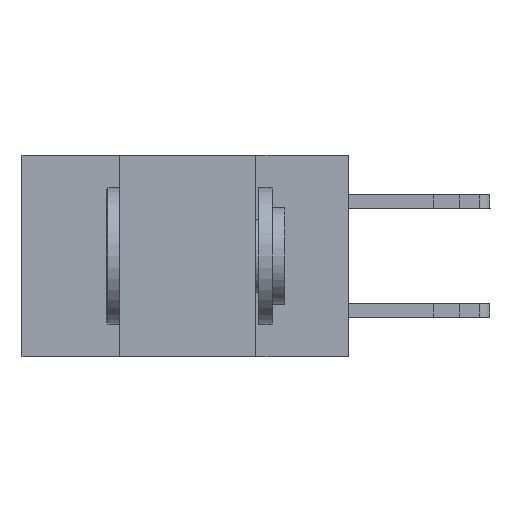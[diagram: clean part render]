
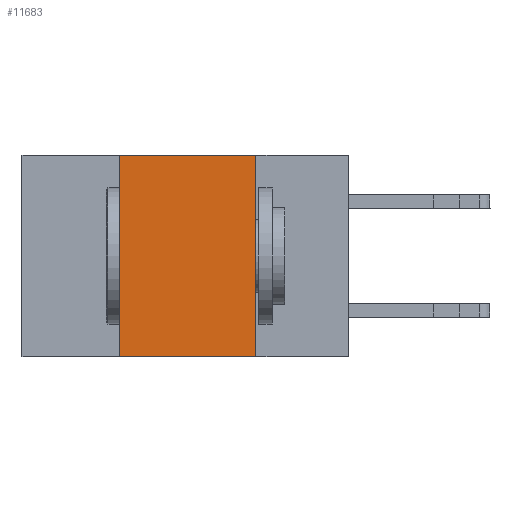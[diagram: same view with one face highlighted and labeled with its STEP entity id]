
A CAD part, left-side view. The second image highlights one B-rep face of the part: STEP entity #11683.
In plain terms, the highlighted planar face has unit normal (-1, 0, 0).
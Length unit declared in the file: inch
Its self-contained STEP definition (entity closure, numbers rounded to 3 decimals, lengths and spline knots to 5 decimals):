
#352 = ORIENTED_EDGE ( 'NONE', *, *, #7029, .T. ) ;
#1140 = CARTESIAN_POINT ( 'NONE',  ( 0., 0.42, -0.37 ) ) ;
#1278 = DIRECTION ( 'NONE',  ( 1., 0., 0. ) ) ;
#1381 = ORIENTED_EDGE ( 'NONE', *, *, #2035, .F. ) ;
#1482 = DIRECTION ( 'NONE',  ( 0., -1., 0. ) ) ;
#1679 = CARTESIAN_POINT ( 'NONE',  ( 0., 0.42, 0. ) ) ;
#1920 = LINE ( 'NONE', #9378, #4436 ) ;
#1985 = DIRECTION ( 'NONE',  ( 0., 0., -1. ) ) ;
#2035 = EDGE_CURVE ( 'NONE', #7792, #5594, #10503, .T. ) ;
#2076 = CARTESIAN_POINT ( 'NONE',  ( 0., 0.17, 0. ) ) ;
#2214 = AXIS2_PLACEMENT_3D ( 'NONE', #6106, #1278, #11693 ) ;
#2642 = VERTEX_POINT ( 'NONE', #2076 ) ;
#3270 = ORIENTED_EDGE ( 'NONE', *, *, #6280, .F. ) ;
#3851 = LINE ( 'NONE', #3910, #9724 ) ;
#3910 = CARTESIAN_POINT ( 'NONE',  ( 0., 0.6, -0.37 ) ) ;
#3925 = VECTOR ( 'NONE', #1482, 39.37008 ) ;
#4041 = EDGE_LOOP ( 'NONE', ( #8827, #3270, #1381, #352 ) ) ;
#4187 = FACE_OUTER_BOUND ( 'NONE', #4041, .T. ) ;
#4194 = LINE ( 'NONE', #5208, #3925 ) ;
#4436 = VECTOR ( 'NONE', #1985, 39.37008 ) ;
#5208 = CARTESIAN_POINT ( 'NONE',  ( 0., 0.6, 0. ) ) ;
#5594 = VERTEX_POINT ( 'NONE', #1679 ) ;
#6106 = CARTESIAN_POINT ( 'NONE',  ( 0., 0.6, 0. ) ) ;
#6280 = EDGE_CURVE ( 'NONE', #5594, #2642, #4194, .T. ) ;
#6944 = VERTEX_POINT ( 'NONE', #10076 ) ;
#7029 = EDGE_CURVE ( 'NONE', #7792, #6944, #3851, .T. ) ;
#7153 = VECTOR ( 'NONE', #8445, 39.37008 ) ;
#7757 = CARTESIAN_POINT ( 'NONE',  ( 0., 0.42, -0.37 ) ) ;
#7792 = VERTEX_POINT ( 'NONE', #1140 ) ;
#8445 = DIRECTION ( 'NONE',  ( 0., 0., 1. ) ) ;
#8827 = ORIENTED_EDGE ( 'NONE', *, *, #11926, .F. ) ;
#9378 = CARTESIAN_POINT ( 'NONE',  ( 0., 0.17, -0.37 ) ) ;
#9724 = VECTOR ( 'NONE', #11361, 39.37008 ) ;
#10076 = CARTESIAN_POINT ( 'NONE',  ( 0., 0.17, -0.37 ) ) ;
#10503 = LINE ( 'NONE', #7757, #7153 ) ;
#10698 = PLANE ( 'NONE',  #2214 ) ;
#11361 = DIRECTION ( 'NONE',  ( 0., -1., 0. ) ) ;
#11683 = ADVANCED_FACE ( 'NONE', ( #4187 ), #10698, .F. ) ;
#11693 = DIRECTION ( 'NONE',  ( 0., 0., -1. ) ) ;
#11926 = EDGE_CURVE ( 'NONE', #2642, #6944, #1920, .T. ) ;
